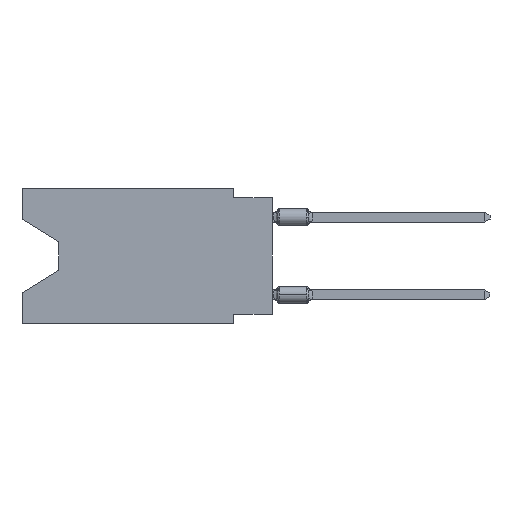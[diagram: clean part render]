
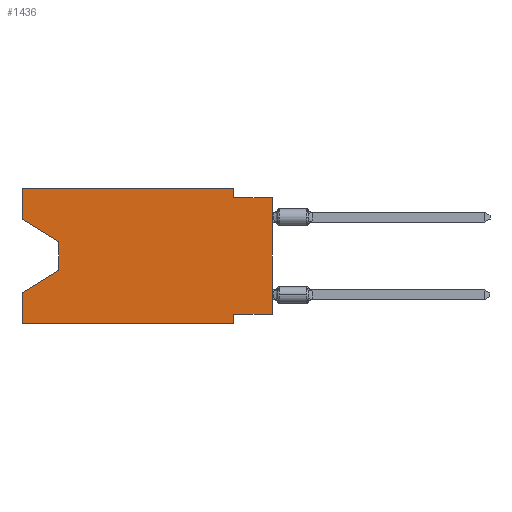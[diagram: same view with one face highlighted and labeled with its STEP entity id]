
A CAD part, left-side view. The second image highlights one B-rep face of the part: STEP entity #1436.
In plain terms, the highlighted planar face has unit normal (-1, 0, 0).
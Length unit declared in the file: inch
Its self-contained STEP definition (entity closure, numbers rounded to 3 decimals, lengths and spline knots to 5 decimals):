
#368 = VERTEX_POINT ( 'NONE', #14020 ) ;
#381 = VECTOR ( 'NONE', #20030, 39.37008 ) ;
#551 = ORIENTED_EDGE ( 'NONE', *, *, #10111, .F. ) ;
#740 = CARTESIAN_POINT ( 'NONE',  ( 0., 0.55, -0.212 ) ) ;
#1038 = VECTOR ( 'NONE', #16075, 39.37008 ) ;
#1388 = CARTESIAN_POINT ( 'NONE',  ( 0., 0.645, 0. ) ) ;
#1436 = ADVANCED_FACE ( 'NONE', ( #7265 ), #23195, .F. ) ;
#1597 = DIRECTION ( 'NONE',  ( 0., -1., 0. ) ) ;
#1663 = DIRECTION ( 'NONE',  ( 0., 0.855, -0.519 ) ) ;
#1889 = ORIENTED_EDGE ( 'NONE', *, *, #26189, .T. ) ;
#2318 = EDGE_LOOP ( 'NONE', ( #16255, #22182, #1889, #551, #20124, #20156, #9205, #5652, #25696, #8206, #21989, #3381 ) ) ;
#2365 = VERTEX_POINT ( 'NONE', #13709 ) ;
#2441 = EDGE_CURVE ( 'NONE', #368, #24127, #22465, .T. ) ;
#2573 = LINE ( 'NONE', #2957, #18997 ) ;
#2957 = CARTESIAN_POINT ( 'NONE',  ( 0., 0., -0.025 ) ) ;
#3367 = VECTOR ( 'NONE', #19709, 39.37008 ) ;
#3381 = ORIENTED_EDGE ( 'NONE', *, *, #21648, .F. ) ;
#3402 = CARTESIAN_POINT ( 'NONE',  ( 0., 0.1, -0.025 ) ) ;
#3819 = CARTESIAN_POINT ( 'NONE',  ( 0., 0.645, 0. ) ) ;
#3877 = DIRECTION ( 'NONE',  ( 0., 0., -1. ) ) ;
#4968 = EDGE_CURVE ( 'NONE', #13546, #2365, #2573, .T. ) ;
#5245 = VECTOR ( 'NONE', #25550, 39.37008 ) ;
#5652 = ORIENTED_EDGE ( 'NONE', *, *, #15246, .T. ) ;
#5673 = VECTOR ( 'NONE', #1663, 39.37008 ) ;
#5735 = CARTESIAN_POINT ( 'NONE',  ( 0., 0.645, 0. ) ) ;
#5757 = CARTESIAN_POINT ( 'NONE',  ( 0., 0., -0.325 ) ) ;
#5824 = CARTESIAN_POINT ( 'NONE',  ( 0., 0.645, -0.35 ) ) ;
#5928 = VERTEX_POINT ( 'NONE', #12368 ) ;
#7265 = FACE_OUTER_BOUND ( 'NONE', #2318, .T. ) ;
#7635 = DIRECTION ( 'NONE',  ( 0., 1., 0. ) ) ;
#7734 = VERTEX_POINT ( 'NONE', #9136 ) ;
#7861 = LINE ( 'NONE', #24204, #1038 ) ;
#8091 = VERTEX_POINT ( 'NONE', #12938 ) ;
#8206 = ORIENTED_EDGE ( 'NONE', *, *, #21225, .F. ) ;
#8628 = CARTESIAN_POINT ( 'NONE',  ( 0., 0.645, -0.08025 ) ) ;
#9085 = LINE ( 'NONE', #25278, #3367 ) ;
#9136 = CARTESIAN_POINT ( 'NONE',  ( 0., 0.1, -0.35 ) ) ;
#9205 = ORIENTED_EDGE ( 'NONE', *, *, #16397, .F. ) ;
#9526 = CARTESIAN_POINT ( 'NONE',  ( 0., 0.55, -0.212 ) ) ;
#9650 = VERTEX_POINT ( 'NONE', #14999 ) ;
#10111 = EDGE_CURVE ( 'NONE', #18612, #8091, #19634, .T. ) ;
#11461 = LINE ( 'NONE', #23570, #13536 ) ;
#12198 = LINE ( 'NONE', #19577, #5245 ) ;
#12368 = CARTESIAN_POINT ( 'NONE',  ( 0., 0.1, 0. ) ) ;
#12705 = AXIS2_PLACEMENT_3D ( 'NONE', #1388, #19474, #12952 ) ;
#12938 = CARTESIAN_POINT ( 'NONE',  ( 0., 0.645, -0.26975 ) ) ;
#12952 = DIRECTION ( 'NONE',  ( 0., 0., -1. ) ) ;
#13425 = VECTOR ( 'NONE', #3877, 39.37008 ) ;
#13453 = DIRECTION ( 'NONE',  ( 0., 0., -1. ) ) ;
#13536 = VECTOR ( 'NONE', #13453, 39.37008 ) ;
#13546 = VERTEX_POINT ( 'NONE', #3402 ) ;
#13675 = VECTOR ( 'NONE', #1597, 39.37008 ) ;
#13709 = CARTESIAN_POINT ( 'NONE',  ( 0., 0., -0.025 ) ) ;
#13918 = DIRECTION ( 'NONE',  ( 0., 0., 1. ) ) ;
#14020 = CARTESIAN_POINT ( 'NONE',  ( 0., 0.55, -0.138 ) ) ;
#14999 = CARTESIAN_POINT ( 'NONE',  ( 0., 0., -0.325 ) ) ;
#15117 = VERTEX_POINT ( 'NONE', #20658 ) ;
#15246 = EDGE_CURVE ( 'NONE', #9650, #2365, #12198, .T. ) ;
#15401 = VERTEX_POINT ( 'NONE', #16985 ) ;
#15694 = LINE ( 'NONE', #5735, #13675 ) ;
#15783 = CARTESIAN_POINT ( 'NONE',  ( 0., 0.645, 0. ) ) ;
#15852 = LINE ( 'NONE', #5757, #17966 ) ;
#16075 = DIRECTION ( 'NONE',  ( 0., 0., -1. ) ) ;
#16255 = ORIENTED_EDGE ( 'NONE', *, *, #20031, .T. ) ;
#16397 = EDGE_CURVE ( 'NONE', #9650, #15117, #15852, .T. ) ;
#16927 = VECTOR ( 'NONE', #22030, 39.37008 ) ;
#16985 = CARTESIAN_POINT ( 'NONE',  ( 0., 0.645, 0. ) ) ;
#17786 = EDGE_CURVE ( 'NONE', #15117, #7734, #7861, .T. ) ;
#17966 = VECTOR ( 'NONE', #7635, 39.37008 ) ;
#18612 = VERTEX_POINT ( 'NONE', #22355 ) ;
#18997 = VECTOR ( 'NONE', #21040, 39.37008 ) ;
#19451 = VERTEX_POINT ( 'NONE', #8628 ) ;
#19474 = DIRECTION ( 'NONE',  ( 1., 0., 0. ) ) ;
#19577 = CARTESIAN_POINT ( 'NONE',  ( 0., 0., 0. ) ) ;
#19634 = LINE ( 'NONE', #3819, #381 ) ;
#19709 = DIRECTION ( 'NONE',  ( 0., -0.855, -0.519 ) ) ;
#19905 = LINE ( 'NONE', #5824, #16927 ) ;
#20030 = DIRECTION ( 'NONE',  ( 0., 0., 1. ) ) ;
#20031 = EDGE_CURVE ( 'NONE', #19451, #368, #9085, .T. ) ;
#20124 = ORIENTED_EDGE ( 'NONE', *, *, #21038, .T. ) ;
#20156 = ORIENTED_EDGE ( 'NONE', *, *, #17786, .F. ) ;
#20161 = LINE ( 'NONE', #15783, #26288 ) ;
#20346 = CARTESIAN_POINT ( 'NONE',  ( 0., 0.55, -0.138 ) ) ;
#20658 = CARTESIAN_POINT ( 'NONE',  ( 0., 0.1, -0.325 ) ) ;
#21038 = EDGE_CURVE ( 'NONE', #18612, #7734, #19905, .T. ) ;
#21040 = DIRECTION ( 'NONE',  ( 0., -1., 0. ) ) ;
#21225 = EDGE_CURVE ( 'NONE', #5928, #13546, #11461, .T. ) ;
#21648 = EDGE_CURVE ( 'NONE', #19451, #15401, #20161, .T. ) ;
#21875 = LINE ( 'NONE', #9526, #5673 ) ;
#21989 = ORIENTED_EDGE ( 'NONE', *, *, #24533, .F. ) ;
#22030 = DIRECTION ( 'NONE',  ( 0., -1., 0. ) ) ;
#22182 = ORIENTED_EDGE ( 'NONE', *, *, #2441, .T. ) ;
#22355 = CARTESIAN_POINT ( 'NONE',  ( 0., 0.645, -0.35 ) ) ;
#22465 = LINE ( 'NONE', #20346, #13425 ) ;
#23195 = PLANE ( 'NONE',  #12705 ) ;
#23570 = CARTESIAN_POINT ( 'NONE',  ( 0., 0.1, 0. ) ) ;
#24127 = VERTEX_POINT ( 'NONE', #740 ) ;
#24204 = CARTESIAN_POINT ( 'NONE',  ( 0., 0.1, -0.35 ) ) ;
#24533 = EDGE_CURVE ( 'NONE', #15401, #5928, #15694, .T. ) ;
#25278 = CARTESIAN_POINT ( 'NONE',  ( 0., 0.645, -0.08025 ) ) ;
#25550 = DIRECTION ( 'NONE',  ( 0., 0., 1. ) ) ;
#25696 = ORIENTED_EDGE ( 'NONE', *, *, #4968, .F. ) ;
#26189 = EDGE_CURVE ( 'NONE', #24127, #8091, #21875, .T. ) ;
#26288 = VECTOR ( 'NONE', #13918, 39.37008 ) ;
